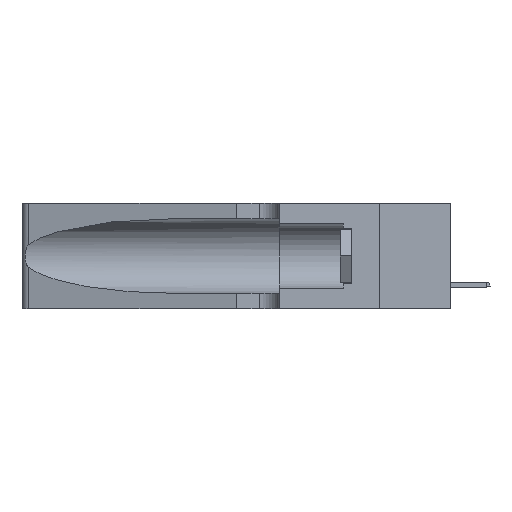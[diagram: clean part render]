
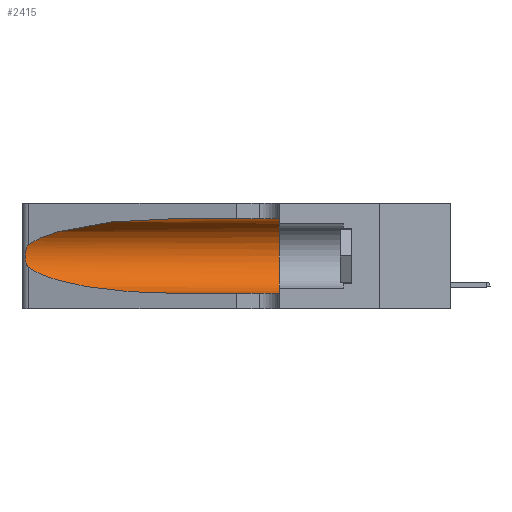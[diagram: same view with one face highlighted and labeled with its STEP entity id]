
A CAD part, left-side view. The second image highlights one B-rep face of the part: STEP entity #2415.
In plain terms, the highlighted cylindrical face has radius 3.308 mm (diameter 6.617 mm), a partial arc.
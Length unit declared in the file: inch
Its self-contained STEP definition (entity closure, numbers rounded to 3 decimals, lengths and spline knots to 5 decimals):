
#808 = DIRECTION ( 'NONE',  ( 0., 0., 1. ) ) ;
#1773 = CARTESIAN_POINT ( 'NONE',  ( 0.25639, 1.23184, 0.21858 ) ) ;
#2247 = CARTESIAN_POINT ( 'NONE',  ( 0.25856, 1.23593, 0.16098 ) ) ;
#2415 = ADVANCED_FACE ( 'NONE', ( #19332 ), #25109, .F. ) ;
#2940 = CARTESIAN_POINT ( 'NONE',  ( 0.26017, 1.23833, 0.17102 ) ) ;
#6039 = CARTESIAN_POINT ( 'NONE',  ( 0.26075, 1.23896, 0.19203 ) ) ;
#6328 = EDGE_CURVE ( 'NONE', #18778, #32573, #38763, .T. ) ;
#6505 = CARTESIAN_POINT ( 'NONE',  ( 0.25555, 1.22993, 0.14849 ) ) ;
#6937 = VERTEX_POINT ( 'NONE', #25680 ) ;
#7102 = CARTESIAN_POINT ( 'NONE',  ( 0.1305, 1.61858, 0.185 ) ) ;
#8097 = ORIENTED_EDGE ( 'NONE', *, *, #6328, .T. ) ;
#8271 = VECTOR ( 'NONE', #27744, 39.37008 ) ;
#10002 = B_SPLINE_CURVE_WITH_KNOTS ( 'NONE', 3,
 ( #44895, #12446, #1773, #34934, #20722, #31376, #6039, #42301, #2940, #2247, #24758, #45825, #6505, #32079 ),
 .UNSPECIFIED., .F., .F.,
 ( 4, 2, 2, 2, 2, 2, 4 ),
 ( 0., 0.00027, 0.00053, 0.00107, 0.0016, 0.00187, 0.00214 ),
 .UNSPECIFIED. ) ;
#12446 = CARTESIAN_POINT ( 'NONE',  ( 0.25555, 1.22994, 0.2215 ) ) ;
#12787 = CARTESIAN_POINT ( 'NONE',  ( 0.2373, 1.15595, 0.08982 ) ) ;
#12999 = EDGE_CURVE ( 'NONE', #25699, #35100, #34636, .T. ) ;
#13348 = AXIS2_PLACEMENT_3D ( 'NONE', #29715, #18830, #808 ) ;
#15650 = CARTESIAN_POINT ( 'NONE',  ( 0.25487, 1.22718, 0.14631 ) ) ;
#15786 =( BOUNDED_CURVE ( )  B_SPLINE_CURVE ( 3, ( #42490, #17154, #34682, #38714 ),
 .UNSPECIFIED., .F., .T. ) 
 B_SPLINE_CURVE_WITH_KNOTS ( ( 4, 4 ),
 ( 1.5708, 2.84003 ),
 .UNSPECIFIED. ) 
 CURVE ( )  GEOMETRIC_REPRESENTATION_ITEM ( )  RATIONAL_B_SPLINE_CURVE ( ( 1., 0.87, 0.87, 1. ) ) 
 REPRESENTATION_ITEM ( '' )  );
#16121 = CARTESIAN_POINT ( 'NONE',  ( 0.25487, 1.22718, 0.14631 ) ) ;
#16616 = EDGE_CURVE ( 'NONE', #32573, #35100, #22279, .T. ) ;
#16627 = LINE ( 'NONE', #20405, #8271 ) ;
#16814 = CARTESIAN_POINT ( 'NONE',  ( 0.18966, 0.96281, 0.05475 ) ) ;
#17154 = CARTESIAN_POINT ( 'NONE',  ( 0.18966, 0.96281, 0.31525 ) ) ;
#18187 = ORIENTED_EDGE ( 'NONE', *, *, #35140, .T. ) ;
#18778 = VERTEX_POINT ( 'NONE', #15650 ) ;
#18830 = DIRECTION ( 'NONE',  ( 0., 1., 0. ) ) ;
#19280 = AXIS2_PLACEMENT_3D ( 'NONE', #7102, #22428, #33567 ) ;
#19332 = FACE_OUTER_BOUND ( 'NONE', #33442, .T. ) ;
#19777 = CARTESIAN_POINT ( 'NONE',  ( 0.1305, 0.35, 0.05475 ) ) ;
#20042 = CARTESIAN_POINT ( 'NONE',  ( 0.1305, 0.72297, 0.05475 ) ) ;
#20405 = CARTESIAN_POINT ( 'NONE',  ( 0.1305, 1.61858, 0.31525 ) ) ;
#20588 = VERTEX_POINT ( 'NONE', #24127 ) ;
#20722 = CARTESIAN_POINT ( 'NONE',  ( 0.25854, 1.2359, 0.20912 ) ) ;
#21685 = ORIENTED_EDGE ( 'NONE', *, *, #31287, .T. ) ;
#21796 = EDGE_CURVE ( 'NONE', #6937, #25699, #16627, .T. ) ;
#22279 = LINE ( 'NONE', #43381, #29986 ) ;
#22428 = DIRECTION ( 'NONE',  ( 0., -1., 0. ) ) ;
#22794 = ORIENTED_EDGE ( 'NONE', *, *, #21796, .F. ) ;
#24127 = CARTESIAN_POINT ( 'NONE',  ( 0.25487, 1.22718, 0.22369 ) ) ;
#24758 = CARTESIAN_POINT ( 'NONE',  ( 0.25789, 1.23486, 0.15765 ) ) ;
#25109 = CYLINDRICAL_SURFACE ( 'NONE', #19280, 0.13025 ) ;
#25680 = CARTESIAN_POINT ( 'NONE',  ( 0.1305, 0.72297, 0.31525 ) ) ;
#25699 = VERTEX_POINT ( 'NONE', #27070 ) ;
#27070 = CARTESIAN_POINT ( 'NONE',  ( 0.1305, 0.35, 0.31525 ) ) ;
#27744 = DIRECTION ( 'NONE',  ( 0., -1., 0. ) ) ;
#29163 = DIRECTION ( 'NONE',  ( 0., -1., 0. ) ) ;
#29715 = CARTESIAN_POINT ( 'NONE',  ( 0.1305, 0.35, 0.185 ) ) ;
#29986 = VECTOR ( 'NONE', #29163, 39.37008 ) ;
#31209 = ORIENTED_EDGE ( 'NONE', *, *, #12999, .F. ) ;
#31287 = EDGE_CURVE ( 'NONE', #6937, #20588, #15786, .T. ) ;
#31376 = CARTESIAN_POINT ( 'NONE',  ( 0.26018, 1.23835, 0.19895 ) ) ;
#32079 = CARTESIAN_POINT ( 'NONE',  ( 0.25487, 1.22718, 0.14631 ) ) ;
#32573 = VERTEX_POINT ( 'NONE', #20042 ) ;
#33012 = ORIENTED_EDGE ( 'NONE', *, *, #16616, .T. ) ;
#33442 = EDGE_LOOP ( 'NONE', ( #21685, #18187, #8097, #33012, #31209, #22794 ) ) ;
#33567 = DIRECTION ( 'NONE',  ( 0., 0., -1. ) ) ;
#34636 = CIRCLE ( 'NONE', #13348, 0.13025 ) ;
#34682 = CARTESIAN_POINT ( 'NONE',  ( 0.2373, 1.15595, 0.28018 ) ) ;
#34934 = CARTESIAN_POINT ( 'NONE',  ( 0.25787, 1.23484, 0.2124 ) ) ;
#35100 = VERTEX_POINT ( 'NONE', #19777 ) ;
#35140 = EDGE_CURVE ( 'NONE', #20588, #18778, #10002, .T. ) ;
#38714 = CARTESIAN_POINT ( 'NONE',  ( 0.25487, 1.22718, 0.22369 ) ) ;
#38763 =( BOUNDED_CURVE ( )  B_SPLINE_CURVE ( 3, ( #16121, #12787, #16814, #45000 ),
 .UNSPECIFIED., .F., .T. ) 
 B_SPLINE_CURVE_WITH_KNOTS ( ( 4, 4 ),
 ( 3.44316, 4.71239 ),
 .UNSPECIFIED. ) 
 CURVE ( )  GEOMETRIC_REPRESENTATION_ITEM ( )  RATIONAL_B_SPLINE_CURVE ( ( 1., 0.87, 0.87, 1. ) ) 
 REPRESENTATION_ITEM ( '' )  );
#42301 = CARTESIAN_POINT ( 'NONE',  ( 0.26075, 1.23896, 0.178 ) ) ;
#42490 = CARTESIAN_POINT ( 'NONE',  ( 0.1305, 0.72297, 0.31525 ) ) ;
#43381 = CARTESIAN_POINT ( 'NONE',  ( 0.1305, 1.61858, 0.05475 ) ) ;
#44895 = CARTESIAN_POINT ( 'NONE',  ( 0.25487, 1.22718, 0.22369 ) ) ;
#45000 = CARTESIAN_POINT ( 'NONE',  ( 0.1305, 0.72297, 0.05475 ) ) ;
#45825 = CARTESIAN_POINT ( 'NONE',  ( 0.25639, 1.23186, 0.15144 ) ) ;
